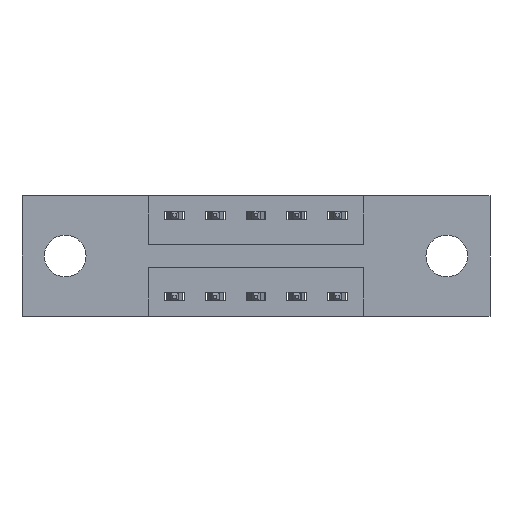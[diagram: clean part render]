
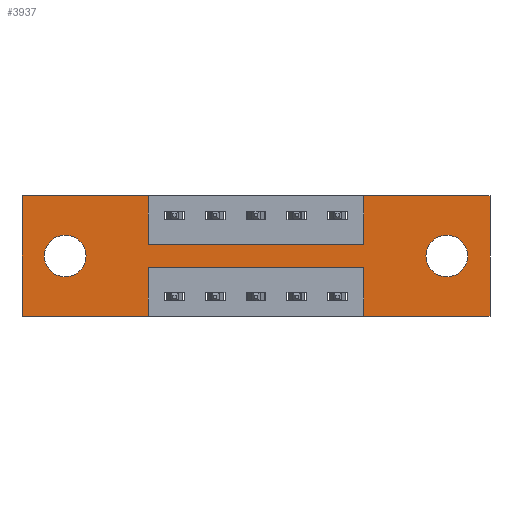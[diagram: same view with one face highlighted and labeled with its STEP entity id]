
A CAD part, front view. The second image highlights one B-rep face of the part: STEP entity #3937.
In plain terms, the highlighted planar face has unit normal (0, -1, 0).
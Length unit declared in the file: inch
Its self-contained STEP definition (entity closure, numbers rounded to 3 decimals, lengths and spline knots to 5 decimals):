
#1 = VERTEX_POINT ( 'NONE', #3945 ) ;
#25 = ORIENTED_EDGE ( 'NONE', *, *, #1599, .F. ) ;
#281 = ORIENTED_EDGE ( 'NONE', *, *, #910, .F. ) ;
#395 = LINE ( 'NONE', #6436, #7788 ) ;
#417 = VERTEX_POINT ( 'NONE', #2452 ) ;
#431 = DIRECTION ( 'NONE',  ( 1., 0., 0. ) ) ;
#460 = AXIS2_PLACEMENT_3D ( 'NONE', #2403, #1219, #574 ) ;
#491 = DIRECTION ( 'NONE',  ( 0., 0., -1. ) ) ;
#509 = EDGE_CURVE ( 'NONE', #5521, #2417, #4093, .T. ) ;
#525 = CARTESIAN_POINT ( 'NONE',  ( 0.3875, 0., -0.15 ) ) ;
#574 = DIRECTION ( 'NONE',  ( 0., 0., -1. ) ) ;
#585 = EDGE_CURVE ( 'NONE', #2586, #2235, #2881, .T. ) ;
#756 = ORIENTED_EDGE ( 'NONE', *, *, #3100, .F. ) ;
#804 = DIRECTION ( 'NONE',  ( 0., 0., -1. ) ) ;
#805 = EDGE_CURVE ( 'NONE', #3534, #1502, #7324, .T. ) ;
#809 = ORIENTED_EDGE ( 'NONE', *, *, #6181, .F. ) ;
#910 = EDGE_CURVE ( 'NONE', #2019, #3667, #3384, .T. ) ;
#929 = DIRECTION ( 'NONE',  ( 0., 0., 1. ) ) ;
#990 = DIRECTION ( 'NONE',  ( 0., 1., 0. ) ) ;
#1026 = DIRECTION ( 'NONE',  ( 0., 0., -1. ) ) ;
#1096 = EDGE_CURVE ( 'NONE', #1, #1127, #4053, .T. ) ;
#1127 = VERTEX_POINT ( 'NONE', #6148 ) ;
#1183 = VERTEX_POINT ( 'NONE', #3469 ) ;
#1191 = VECTOR ( 'NONE', #7773, 39.37008 ) ;
#1204 = CIRCLE ( 'NONE', #4978, 0.064 ) ;
#1219 = DIRECTION ( 'NONE',  ( 0., -1., 0. ) ) ;
#1263 = CARTESIAN_POINT ( 'NONE',  ( 0., 0., 0. ) ) ;
#1282 = LINE ( 'NONE', #6229, #7621 ) ;
#1304 = EDGE_CURVE ( 'NONE', #2235, #417, #6916, .T. ) ;
#1322 = EDGE_CURVE ( 'NONE', #1968, #2255, #395, .T. ) ;
#1343 = CARTESIAN_POINT ( 'NONE',  ( 0., 0., -0.37 ) ) ;
#1460 = LINE ( 'NONE', #2257, #4821 ) ;
#1502 = VERTEX_POINT ( 'NONE', #3236 ) ;
#1546 = DIRECTION ( 'NONE',  ( 0., 0., 1. ) ) ;
#1599 = EDGE_CURVE ( 'NONE', #2255, #2019, #6216, .T. ) ;
#1611 = LINE ( 'NONE', #8150, #5883 ) ;
#1780 = EDGE_LOOP ( 'NONE', ( #6797, #5417 ) ) ;
#1821 = CARTESIAN_POINT ( 'NONE',  ( 0.3875, 0., 0. ) ) ;
#1968 = VERTEX_POINT ( 'NONE', #5840 ) ;
#2019 = VERTEX_POINT ( 'NONE', #2137 ) ;
#2034 = EDGE_CURVE ( 'NONE', #2417, #5521, #1204, .T. ) ;
#2109 = EDGE_CURVE ( 'NONE', #4022, #3534, #3707, .T. ) ;
#2137 = CARTESIAN_POINT ( 'NONE',  ( 1.0475, 0., -0.37 ) ) ;
#2235 = VERTEX_POINT ( 'NONE', #1343 ) ;
#2255 = VERTEX_POINT ( 'NONE', #7030 ) ;
#2257 = CARTESIAN_POINT ( 'NONE',  ( 1.0475, 0., 0. ) ) ;
#2354 = LINE ( 'NONE', #7844, #4801 ) ;
#2403 = CARTESIAN_POINT ( 'NONE',  ( 0., 0., -0.37 ) ) ;
#2417 = VERTEX_POINT ( 'NONE', #2922 ) ;
#2419 = AXIS2_PLACEMENT_3D ( 'NONE', #4602, #2751, #3356 ) ;
#2452 = CARTESIAN_POINT ( 'NONE',  ( 0., 0., 0. ) ) ;
#2506 = ORIENTED_EDGE ( 'NONE', *, *, #585, .F. ) ;
#2586 = VERTEX_POINT ( 'NONE', #6755 ) ;
#2751 = DIRECTION ( 'NONE',  ( 0., 1., 0. ) ) ;
#2762 = EDGE_CURVE ( 'NONE', #5083, #2586, #1282, .T. ) ;
#2881 = LINE ( 'NONE', #6092, #5152 ) ;
#2922 = CARTESIAN_POINT ( 'NONE',  ( 1.3025, 0., -0.121 ) ) ;
#3100 = EDGE_CURVE ( 'NONE', #1502, #1183, #1460, .T. ) ;
#3174 = EDGE_LOOP ( 'NONE', ( #7501, #7834 ) ) ;
#3202 = ORIENTED_EDGE ( 'NONE', *, *, #2109, .F. ) ;
#3236 = CARTESIAN_POINT ( 'NONE',  ( 1.0475, 0., -0.15 ) ) ;
#3356 = DIRECTION ( 'NONE',  ( 0., 0., -1. ) ) ;
#3384 = LINE ( 'NONE', #5666, #4068 ) ;
#3406 = CARTESIAN_POINT ( 'NONE',  ( 1.0475, 0., -0.22 ) ) ;
#3469 = CARTESIAN_POINT ( 'NONE',  ( 1.0475, 0., 0. ) ) ;
#3534 = VERTEX_POINT ( 'NONE', #6421 ) ;
#3667 = VERTEX_POINT ( 'NONE', #3406 ) ;
#3684 = PLANE ( 'NONE',  #460 ) ;
#3707 = LINE ( 'NONE', #8117, #6668 ) ;
#3750 = ORIENTED_EDGE ( 'NONE', *, *, #1322, .F. ) ;
#3776 = DIRECTION ( 'NONE',  ( 1., 0., 0. ) ) ;
#3937 = ADVANCED_FACE ( 'NONE', ( #6073, #6858, #4747 ), #3684, .T. ) ;
#3945 = CARTESIAN_POINT ( 'NONE',  ( 0.1325, 0., -0.121 ) ) ;
#4022 = VERTEX_POINT ( 'NONE', #1821 ) ;
#4053 = CIRCLE ( 'NONE', #7386, 0.064 ) ;
#4061 = CARTESIAN_POINT ( 'NONE',  ( 0., 0., 0. ) ) ;
#4068 = VECTOR ( 'NONE', #5695, 39.37008 ) ;
#4093 = CIRCLE ( 'NONE', #2419, 0.064 ) ;
#4185 = ORIENTED_EDGE ( 'NONE', *, *, #8062, .F. ) ;
#4339 = VECTOR ( 'NONE', #6323, 39.37008 ) ;
#4546 = ORIENTED_EDGE ( 'NONE', *, *, #805, .F. ) ;
#4602 = CARTESIAN_POINT ( 'NONE',  ( 1.3025, 0., -0.185 ) ) ;
#4611 = ORIENTED_EDGE ( 'NONE', *, *, #7269, .F. ) ;
#4705 = CARTESIAN_POINT ( 'NONE',  ( 0.1325, 0., -0.185 ) ) ;
#4747 = FACE_OUTER_BOUND ( 'NONE', #7209, .T. ) ;
#4801 = VECTOR ( 'NONE', #7820, 39.37008 ) ;
#4821 = VECTOR ( 'NONE', #1546, 39.37008 ) ;
#4843 = CARTESIAN_POINT ( 'NONE',  ( 0.1325, 0., -0.185 ) ) ;
#4925 = DIRECTION ( 'NONE',  ( 0., 0., -1. ) ) ;
#4978 = AXIS2_PLACEMENT_3D ( 'NONE', #6720, #7816, #1026 ) ;
#4985 = DIRECTION ( 'NONE',  ( -1., 0., 0. ) ) ;
#5001 = CARTESIAN_POINT ( 'NONE',  ( 1.3025, 0., -0.249 ) ) ;
#5038 = LINE ( 'NONE', #4061, #1191 ) ;
#5083 = VERTEX_POINT ( 'NONE', #6329 ) ;
#5152 = VECTOR ( 'NONE', #6709, 39.37008 ) ;
#5417 = ORIENTED_EDGE ( 'NONE', *, *, #509, .T. ) ;
#5483 = DIRECTION ( 'NONE',  ( 0., 1., 0. ) ) ;
#5487 = ORIENTED_EDGE ( 'NONE', *, *, #1304, .F. ) ;
#5521 = VERTEX_POINT ( 'NONE', #5001 ) ;
#5558 = DIRECTION ( 'NONE',  ( 0., 0., 1. ) ) ;
#5663 = CARTESIAN_POINT ( 'NONE',  ( 0., 0., -0.37 ) ) ;
#5666 = CARTESIAN_POINT ( 'NONE',  ( 1.0475, 0., -0.37 ) ) ;
#5695 = DIRECTION ( 'NONE',  ( 0., 0., 1. ) ) ;
#5765 = CIRCLE ( 'NONE', #7579, 0.064 ) ;
#5840 = CARTESIAN_POINT ( 'NONE',  ( 1.435, 0., 0. ) ) ;
#5883 = VECTOR ( 'NONE', #3776, 39.37008 ) ;
#6031 = VECTOR ( 'NONE', #4985, 39.37008 ) ;
#6073 = FACE_BOUND ( 'NONE', #1780, .T. ) ;
#6092 = CARTESIAN_POINT ( 'NONE',  ( 0., 0., -0.37 ) ) ;
#6148 = CARTESIAN_POINT ( 'NONE',  ( 0.1325, 0., -0.249 ) ) ;
#6181 = EDGE_CURVE ( 'NONE', #3667, #5083, #2354, .T. ) ;
#6216 = LINE ( 'NONE', #5663, #6031 ) ;
#6229 = CARTESIAN_POINT ( 'NONE',  ( 0.3875, 0., -0.37 ) ) ;
#6323 = DIRECTION ( 'NONE',  ( 0., 0., 1. ) ) ;
#6329 = CARTESIAN_POINT ( 'NONE',  ( 0.3875, 0., -0.22 ) ) ;
#6345 = VECTOR ( 'NONE', #431, 39.37008 ) ;
#6421 = CARTESIAN_POINT ( 'NONE',  ( 0.3875, 0., -0.15 ) ) ;
#6436 = CARTESIAN_POINT ( 'NONE',  ( 1.435, 0., 0. ) ) ;
#6668 = VECTOR ( 'NONE', #4925, 39.37008 ) ;
#6709 = DIRECTION ( 'NONE',  ( -1., 0., 0. ) ) ;
#6720 = CARTESIAN_POINT ( 'NONE',  ( 1.3025, 0., -0.185 ) ) ;
#6755 = CARTESIAN_POINT ( 'NONE',  ( 0.3875, 0., -0.37 ) ) ;
#6797 = ORIENTED_EDGE ( 'NONE', *, *, #2034, .T. ) ;
#6803 = EDGE_CURVE ( 'NONE', #1127, #1, #5765, .T. ) ;
#6858 = FACE_BOUND ( 'NONE', #3174, .T. ) ;
#6916 = LINE ( 'NONE', #1263, #4339 ) ;
#7030 = CARTESIAN_POINT ( 'NONE',  ( 1.435, 0., -0.37 ) ) ;
#7209 = EDGE_LOOP ( 'NONE', ( #7376, #809, #281, #25, #3750, #4185, #756, #4546, #3202, #4611, #5487, #2506 ) ) ;
#7269 = EDGE_CURVE ( 'NONE', #417, #4022, #5038, .T. ) ;
#7324 = LINE ( 'NONE', #525, #6345 ) ;
#7376 = ORIENTED_EDGE ( 'NONE', *, *, #2762, .F. ) ;
#7386 = AXIS2_PLACEMENT_3D ( 'NONE', #4843, #5483, #5558 ) ;
#7501 = ORIENTED_EDGE ( 'NONE', *, *, #1096, .T. ) ;
#7579 = AXIS2_PLACEMENT_3D ( 'NONE', #4705, #990, #929 ) ;
#7621 = VECTOR ( 'NONE', #491, 39.37008 ) ;
#7773 = DIRECTION ( 'NONE',  ( 1., 0., 0. ) ) ;
#7788 = VECTOR ( 'NONE', #804, 39.37008 ) ;
#7816 = DIRECTION ( 'NONE',  ( 0., 1., 0. ) ) ;
#7820 = DIRECTION ( 'NONE',  ( -1., 0., 0. ) ) ;
#7834 = ORIENTED_EDGE ( 'NONE', *, *, #6803, .T. ) ;
#7844 = CARTESIAN_POINT ( 'NONE',  ( 0.3875, 0., -0.22 ) ) ;
#8062 = EDGE_CURVE ( 'NONE', #1183, #1968, #1611, .T. ) ;
#8117 = CARTESIAN_POINT ( 'NONE',  ( 0.3875, 0., 0. ) ) ;
#8150 = CARTESIAN_POINT ( 'NONE',  ( 0., 0., 0. ) ) ;
